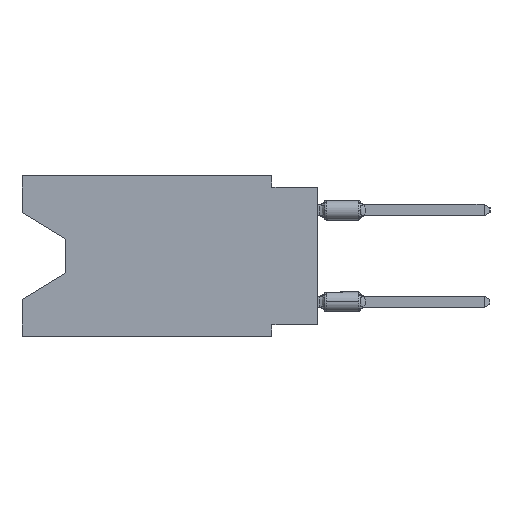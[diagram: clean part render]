
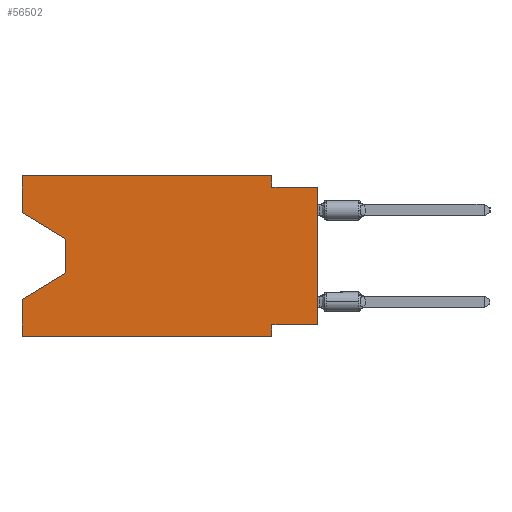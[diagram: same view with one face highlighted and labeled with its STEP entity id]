
A CAD part, left-side view. The second image highlights one B-rep face of the part: STEP entity #56502.
In plain terms, the highlighted planar face has unit normal (-1, 0, 0).
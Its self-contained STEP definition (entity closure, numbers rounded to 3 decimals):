
#1507 = DIRECTION ( 'NONE',  ( 0., 0., 1. ) ) ;
#2161 = EDGE_CURVE ( 'NONE', #14422, #24213, #25896, .T. ) ;
#3381 = LINE ( 'NONE', #26230, #48976 ) ;
#3404 = ORIENTED_EDGE ( 'NONE', *, *, #36714, .F. ) ;
#3527 = VECTOR ( 'NONE', #25340, 1000. ) ;
#4746 = VERTEX_POINT ( 'NONE', #9616 ) ;
#4800 = PLANE ( 'NONE',  #54141 ) ;
#5394 = EDGE_CURVE ( 'NONE', #37148, #57854, #16732, .T. ) ;
#5827 = VECTOR ( 'NONE', #28049, 1000. ) ;
#6213 = CARTESIAN_POINT ( 'NONE',  ( 0., 16.383, 0. ) ) ;
#6235 = DIRECTION ( 'NONE',  ( 0., -1., 0. ) ) ;
#6990 = LINE ( 'NONE', #16901, #58024 ) ;
#8171 = VERTEX_POINT ( 'NONE', #17076 ) ;
#8348 = ORIENTED_EDGE ( 'NONE', *, *, #2161, .T. ) ;
#8916 = CARTESIAN_POINT ( 'NONE',  ( 0., 13.97, -5.385 ) ) ;
#9210 = LINE ( 'NONE', #8916, #46693 ) ;
#9616 = CARTESIAN_POINT ( 'NONE',  ( 0., 13.97, -5.385 ) ) ;
#9989 = ORIENTED_EDGE ( 'NONE', *, *, #44128, .T. ) ;
#10240 = VECTOR ( 'NONE', #54203, 1000. ) ;
#12010 = VECTOR ( 'NONE', #58731, 1000. ) ;
#12069 = CARTESIAN_POINT ( 'NONE',  ( 0., 16.383, -2.038 ) ) ;
#13021 = ORIENTED_EDGE ( 'NONE', *, *, #14844, .T. ) ;
#13447 = VERTEX_POINT ( 'NONE', #55151 ) ;
#13516 = DIRECTION ( 'NONE',  ( 0., 0., -1. ) ) ;
#14422 = VERTEX_POINT ( 'NONE', #40874 ) ;
#14676 = VECTOR ( 'NONE', #6235, 1000. ) ;
#14844 = EDGE_CURVE ( 'NONE', #4746, #33420, #9210, .T. ) ;
#15261 = LINE ( 'NONE', #42605, #14676 ) ;
#15705 = EDGE_CURVE ( 'NONE', #57854, #13447, #49092, .T. ) ;
#16732 = LINE ( 'NONE', #34176, #48227 ) ;
#16901 = CARTESIAN_POINT ( 'NONE',  ( 0., 0., 0. ) ) ;
#17076 = CARTESIAN_POINT ( 'NONE',  ( 0., 16.383, -8.89 ) ) ;
#17646 = DIRECTION ( 'NONE',  ( 0., 0.855, -0.519 ) ) ;
#18399 = LINE ( 'NONE', #35869, #10240 ) ;
#20131 = CARTESIAN_POINT ( 'NONE',  ( 0., 2.54, 0. ) ) ;
#20152 = ORIENTED_EDGE ( 'NONE', *, *, #25912, .F. ) ;
#20226 = LINE ( 'NONE', #38568, #5827 ) ;
#21726 = CARTESIAN_POINT ( 'NONE',  ( 0., 2.54, 0. ) ) ;
#22453 = EDGE_CURVE ( 'NONE', #47091, #56950, #6990, .T. ) ;
#23321 = CARTESIAN_POINT ( 'NONE',  ( 0., 13.97, -3.505 ) ) ;
#23346 = ORIENTED_EDGE ( 'NONE', *, *, #23430, .F. ) ;
#23430 = EDGE_CURVE ( 'NONE', #8171, #33420, #28872, .T. ) ;
#24213 = VERTEX_POINT ( 'NONE', #50010 ) ;
#24371 = EDGE_LOOP ( 'NONE', ( #8348, #25056, #13021, #23346, #9989, #20152, #49187, #36456, #51424, #57968, #30337, #3404 ) ) ;
#24860 = CARTESIAN_POINT ( 'NONE',  ( 0., 16.383, 0. ) ) ;
#25056 = ORIENTED_EDGE ( 'NONE', *, *, #45886, .T. ) ;
#25340 = DIRECTION ( 'NONE',  ( 0., 0., -1. ) ) ;
#25896 = LINE ( 'NONE', #12069, #25971 ) ;
#25912 = EDGE_CURVE ( 'NONE', #45169, #44898, #20226, .T. ) ;
#25971 = VECTOR ( 'NONE', #43623, 1000. ) ;
#26230 = CARTESIAN_POINT ( 'NONE',  ( 0., 0., -0.635 ) ) ;
#26511 = DIRECTION ( 'NONE',  ( 0., 0., 1. ) ) ;
#26562 = CARTESIAN_POINT ( 'NONE',  ( 0., 2.54, -8.89 ) ) ;
#28049 = DIRECTION ( 'NONE',  ( 0., 0., -1. ) ) ;
#28872 = LINE ( 'NONE', #47502, #44610 ) ;
#30337 = ORIENTED_EDGE ( 'NONE', *, *, #5394, .F. ) ;
#33420 = VERTEX_POINT ( 'NONE', #49705 ) ;
#33424 = EDGE_CURVE ( 'NONE', #47091, #45169, #35591, .T. ) ;
#34176 = CARTESIAN_POINT ( 'NONE',  ( 0., 16.383, 0. ) ) ;
#35591 = LINE ( 'NONE', #54506, #12010 ) ;
#35869 = CARTESIAN_POINT ( 'NONE',  ( 0., 16.383, 0. ) ) ;
#36456 = ORIENTED_EDGE ( 'NONE', *, *, #22453, .T. ) ;
#36714 = EDGE_CURVE ( 'NONE', #14422, #37148, #18399, .T. ) ;
#37148 = VERTEX_POINT ( 'NONE', #24860 ) ;
#37956 = VECTOR ( 'NONE', #41648, 1000. ) ;
#38340 = LINE ( 'NONE', #23321, #37956 ) ;
#38568 = CARTESIAN_POINT ( 'NONE',  ( 0., 2.54, -8.89 ) ) ;
#40874 = CARTESIAN_POINT ( 'NONE',  ( 0., 16.383, -2.038 ) ) ;
#40965 = EDGE_CURVE ( 'NONE', #13447, #56950, #3381, .T. ) ;
#41648 = DIRECTION ( 'NONE',  ( 0., 0., -1. ) ) ;
#42605 = CARTESIAN_POINT ( 'NONE',  ( 0., 16.383, -8.89 ) ) ;
#43623 = DIRECTION ( 'NONE',  ( 0., -0.855, -0.519 ) ) ;
#44128 = EDGE_CURVE ( 'NONE', #8171, #44898, #15261, .T. ) ;
#44557 = DIRECTION ( 'NONE',  ( 0., -1., 0. ) ) ;
#44610 = VECTOR ( 'NONE', #1507, 1000. ) ;
#44898 = VERTEX_POINT ( 'NONE', #26562 ) ;
#45169 = VERTEX_POINT ( 'NONE', #49798 ) ;
#45886 = EDGE_CURVE ( 'NONE', #24213, #4746, #38340, .T. ) ;
#46693 = VECTOR ( 'NONE', #17646, 1000. ) ;
#46767 = CARTESIAN_POINT ( 'NONE',  ( 0., 0., -8.255 ) ) ;
#47091 = VERTEX_POINT ( 'NONE', #46767 ) ;
#47502 = CARTESIAN_POINT ( 'NONE',  ( 0., 16.383, 0. ) ) ;
#48227 = VECTOR ( 'NONE', #52512, 1000. ) ;
#48976 = VECTOR ( 'NONE', #44557, 1000. ) ;
#49092 = LINE ( 'NONE', #21726, #3527 ) ;
#49187 = ORIENTED_EDGE ( 'NONE', *, *, #33424, .F. ) ;
#49705 = CARTESIAN_POINT ( 'NONE',  ( 0., 16.383, -6.852 ) ) ;
#49798 = CARTESIAN_POINT ( 'NONE',  ( 0., 2.54, -8.255 ) ) ;
#50010 = CARTESIAN_POINT ( 'NONE',  ( 0., 13.97, -3.505 ) ) ;
#50206 = FACE_OUTER_BOUND ( 'NONE', #24371, .T. ) ;
#51236 = CARTESIAN_POINT ( 'NONE',  ( 0., 0., -0.635 ) ) ;
#51424 = ORIENTED_EDGE ( 'NONE', *, *, #40965, .F. ) ;
#52512 = DIRECTION ( 'NONE',  ( 0., -1., 0. ) ) ;
#54141 = AXIS2_PLACEMENT_3D ( 'NONE', #6213, #54709, #13516 ) ;
#54203 = DIRECTION ( 'NONE',  ( 0., 0., 1. ) ) ;
#54506 = CARTESIAN_POINT ( 'NONE',  ( 0., 0., -8.255 ) ) ;
#54709 = DIRECTION ( 'NONE',  ( 1., 0., 0. ) ) ;
#55151 = CARTESIAN_POINT ( 'NONE',  ( 0., 2.54, -0.635 ) ) ;
#56502 = ADVANCED_FACE ( 'NONE', ( #50206 ), #4800, .F. ) ;
#56950 = VERTEX_POINT ( 'NONE', #51236 ) ;
#57854 = VERTEX_POINT ( 'NONE', #20131 ) ;
#57968 = ORIENTED_EDGE ( 'NONE', *, *, #15705, .F. ) ;
#58024 = VECTOR ( 'NONE', #26511, 1000. ) ;
#58731 = DIRECTION ( 'NONE',  ( 0., 1., 0. ) ) ;
